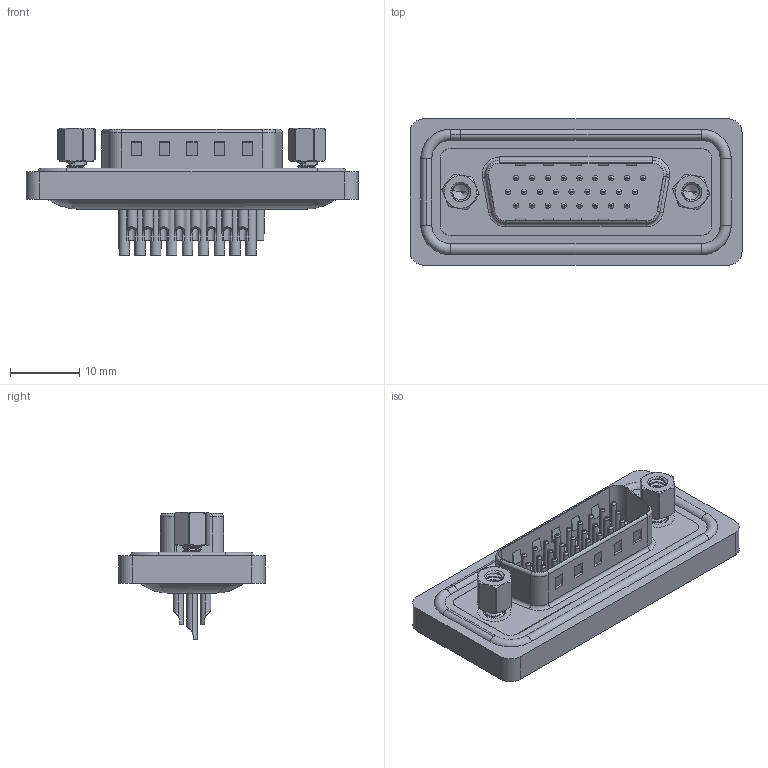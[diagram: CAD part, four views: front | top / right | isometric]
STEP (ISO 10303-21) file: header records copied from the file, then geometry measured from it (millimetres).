
FILE_DESCRIPTION (( 'STEP AP203' ), '1' );
FILE_NAME ('637-W26-622-012.STEP', '2024-04-12T19:55:00', ( '' ), ( '' ), 'SwSTEP 2.0', 'SolidWorks 2023', '' );
FILE_SCHEMA (( 'CONFIG_CONTROL_DESIGN' ));
Length unit declared in the file: millimetre
Products named in the file (9): 637W Contact Row 3_22; 637W Waterproof Housing_26 Contacts; 637W Contact Row 2_22; 637W Contact Row 1_22; 637W 4-40 Hex Standoff; 637-W26-622-012; 637W Housing_26 Contacts; 637W 4-40 Threaded Rivet; 637W Shell_26 Contacts
Assembly tree (33 placements, depth 2):
  637-W26-622-012
    637W Housing_26 Contacts
    637W Shell_26 Contacts
    637W Contact Row 1_22  x9
    637W Contact Row 2_22  x9
    637W Contact Row 3_22  x8
    637W Waterproof Housing_26 Contacts
    637W 4-40 Threaded Rivet  x2
    637W 4-40 Hex Standoff  x2
Bounding box: 47.89 x 21.1 x 18.45 mm (x, y, z)
Volume: 4968.4 mm3; surface area: 9096.5 mm2
Topology: 34 solids, 34 shells, 1498 faces, 3592 edges, 2225 vertices
Faces by surface type: cylinder 684, plane 407, torus 303, cone 82, bspline 22
Entity records: 27847 total; most frequent: CARTESIAN_POINT 8190, DIRECTION 3979, ORIENTED_EDGE 3612, EDGE_CURVE 1806, AXIS2_PLACEMENT_3D 1590, VERTEX_POINT 1163, EDGE_LOOP 941, CIRCLE 833
